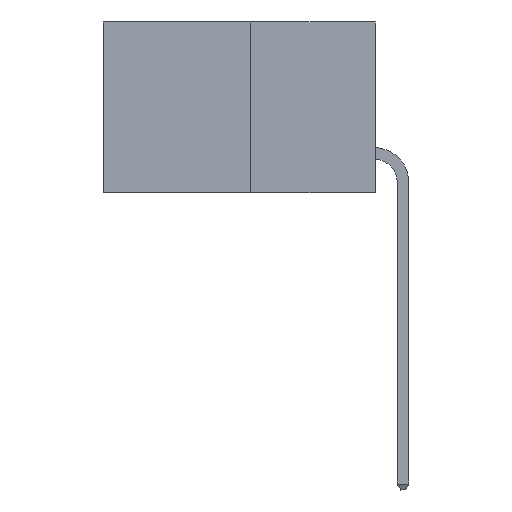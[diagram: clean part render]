
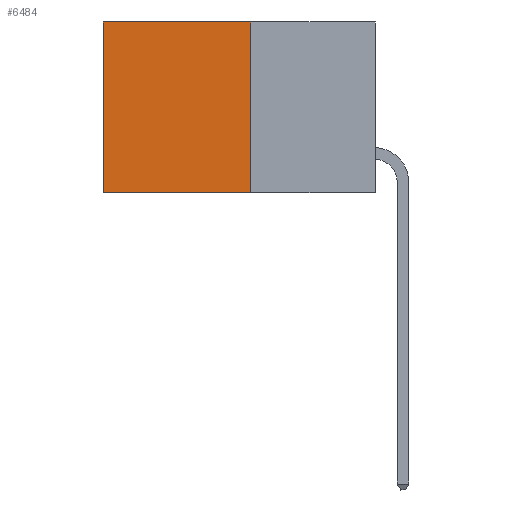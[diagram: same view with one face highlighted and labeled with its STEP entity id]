
A CAD part, left-side view. The second image highlights one B-rep face of the part: STEP entity #6484.
In plain terms, the highlighted planar face has unit normal (-1, 0, 0).
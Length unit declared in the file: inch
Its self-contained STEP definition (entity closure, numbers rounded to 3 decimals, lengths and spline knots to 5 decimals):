
#268 = AXIS2_PLACEMENT_3D ( 'NONE', #6806, #648, #7755 ) ;
#360 = CARTESIAN_POINT ( 'NONE',  ( 0.277, 0.27, -0.37 ) ) ;
#525 = CARTESIAN_POINT ( 'NONE',  ( 0.277, 0.27, -0.37 ) ) ;
#648 = DIRECTION ( 'NONE',  ( 1., 0., 0. ) ) ;
#1499 = EDGE_CURVE ( 'NONE', #9893, #10512, #10786, .T. ) ;
#1545 = LINE ( 'NONE', #4765, #6600 ) ;
#2171 = LINE ( 'NONE', #525, #4585 ) ;
#2551 = CARTESIAN_POINT ( 'NONE',  ( 0.277, 0.27, 0. ) ) ;
#3948 = EDGE_CURVE ( 'NONE', #10512, #10299, #1545, .T. ) ;
#4000 = DIRECTION ( 'NONE',  ( 0., 1., 0. ) ) ;
#4128 = ORIENTED_EDGE ( 'NONE', *, *, #3948, .T. ) ;
#4173 = ORIENTED_EDGE ( 'NONE', *, *, #10003, .F. ) ;
#4231 = LINE ( 'NONE', #4420, #9009 ) ;
#4353 = ORIENTED_EDGE ( 'NONE', *, *, #11726, .F. ) ;
#4368 = ORIENTED_EDGE ( 'NONE', *, *, #1499, .T. ) ;
#4420 = CARTESIAN_POINT ( 'NONE',  ( 0.277, 0.27, -0.37 ) ) ;
#4585 = VECTOR ( 'NONE', #5632, 39.37008 ) ;
#4765 = CARTESIAN_POINT ( 'NONE',  ( 0.277, 0.59, -0.37 ) ) ;
#5632 = DIRECTION ( 'NONE',  ( 0., 1., 0. ) ) ;
#5803 = PLANE ( 'NONE',  #268 ) ;
#5903 = EDGE_LOOP ( 'NONE', ( #4128, #4173, #4353, #4368 ) ) ;
#6117 = DIRECTION ( 'NONE',  ( 0., 0., -1. ) ) ;
#6484 = ADVANCED_FACE ( 'NONE', ( #9850 ), #5803, .F. ) ;
#6600 = VECTOR ( 'NONE', #6117, 39.37008 ) ;
#6806 = CARTESIAN_POINT ( 'NONE',  ( 0.277, 0.27, -0.37 ) ) ;
#7311 = DIRECTION ( 'NONE',  ( 0., 0., -1. ) ) ;
#7755 = DIRECTION ( 'NONE',  ( 0., 0., -1. ) ) ;
#7975 = CARTESIAN_POINT ( 'NONE',  ( 0.277, 0.59, -0.37 ) ) ;
#8003 = VERTEX_POINT ( 'NONE', #360 ) ;
#8990 = VECTOR ( 'NONE', #4000, 39.37008 ) ;
#9009 = VECTOR ( 'NONE', #7311, 39.37008 ) ;
#9292 = CARTESIAN_POINT ( 'NONE',  ( 0.277, 0.27, 0. ) ) ;
#9850 = FACE_OUTER_BOUND ( 'NONE', #5903, .T. ) ;
#9893 = VERTEX_POINT ( 'NONE', #2551 ) ;
#10003 = EDGE_CURVE ( 'NONE', #8003, #10299, #2171, .T. ) ;
#10299 = VERTEX_POINT ( 'NONE', #7975 ) ;
#10512 = VERTEX_POINT ( 'NONE', #10887 ) ;
#10786 = LINE ( 'NONE', #9292, #8990 ) ;
#10887 = CARTESIAN_POINT ( 'NONE',  ( 0.277, 0.59, 0. ) ) ;
#11726 = EDGE_CURVE ( 'NONE', #9893, #8003, #4231, .T. ) ;
